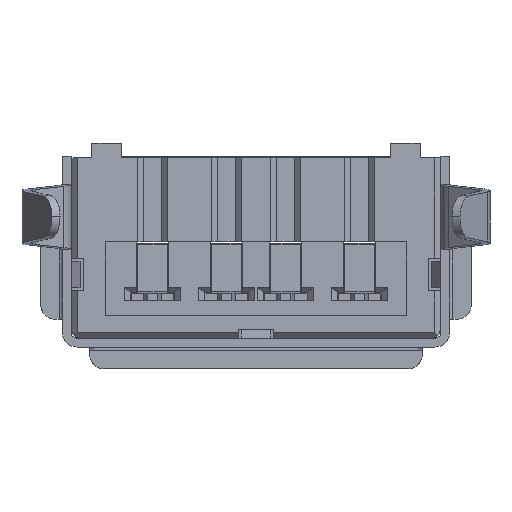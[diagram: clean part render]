
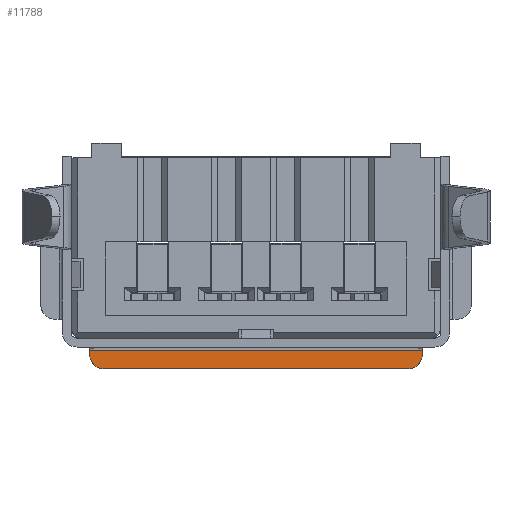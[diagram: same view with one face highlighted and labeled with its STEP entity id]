
A CAD part, front view. The second image highlights one B-rep face of the part: STEP entity #11788.
In plain terms, the highlighted planar face has unit normal (0, -1, 0).
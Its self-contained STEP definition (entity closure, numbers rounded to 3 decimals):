
#174 = CARTESIAN_POINT ( 'NONE',  ( 5.625, 6.85, 0. ) ) ;
#301 = VECTOR ( 'NONE', #9829, 1000. ) ;
#624 = VECTOR ( 'NONE', #3200, 1000. ) ;
#785 = AXIS2_PLACEMENT_3D ( 'NONE', #11261, #17445, #7973 ) ;
#992 = VERTEX_POINT ( 'NONE', #19504 ) ;
#1148 = CARTESIAN_POINT ( 'NONE',  ( -5.625, 6.85, -0.4 ) ) ;
#2433 = AXIS2_PLACEMENT_3D ( 'NONE', #8808, #13946, #12000 ) ;
#2630 = VERTEX_POINT ( 'NONE', #15059 ) ;
#3095 = LINE ( 'NONE', #17503, #624 ) ;
#3200 = DIRECTION ( 'NONE',  ( 1., 0., 0. ) ) ;
#3764 = CIRCLE ( 'NONE', #17918, 0.5 ) ;
#3880 = VECTOR ( 'NONE', #15398, 1000. ) ;
#4156 = ORIENTED_EDGE ( 'NONE', *, *, #19806, .T. ) ;
#4243 = EDGE_CURVE ( 'NONE', #11407, #992, #13577, .T. ) ;
#4872 = VERTEX_POINT ( 'NONE', #6754 ) ;
#5032 = DIRECTION ( 'NONE',  ( 0., -1., 0. ) ) ;
#5617 = EDGE_CURVE ( 'NONE', #4872, #19357, #3095, .T. ) ;
#5754 = DIRECTION ( 'NONE',  ( 0., 0., -1. ) ) ;
#5923 = VERTEX_POINT ( 'NONE', #6141 ) ;
#6001 = EDGE_CURVE ( 'NONE', #5923, #2630, #6344, .T. ) ;
#6004 = ORIENTED_EDGE ( 'NONE', *, *, #12941, .T. ) ;
#6141 = CARTESIAN_POINT ( 'NONE',  ( 5.625, 6.85, -0.54 ) ) ;
#6344 = LINE ( 'NONE', #174, #301 ) ;
#6754 = CARTESIAN_POINT ( 'NONE',  ( -5.125, 6.85, -1.04 ) ) ;
#7274 = PLANE ( 'NONE',  #2433 ) ;
#7476 = LINE ( 'NONE', #13750, #3880 ) ;
#7679 = CIRCLE ( 'NONE', #785, 0.5 ) ;
#7973 = DIRECTION ( 'NONE',  ( 0., 0., -1. ) ) ;
#8808 = CARTESIAN_POINT ( 'NONE',  ( 0., 6.85, 0. ) ) ;
#8952 = EDGE_CURVE ( 'NONE', #19357, #5923, #3764, .T. ) ;
#9829 = DIRECTION ( 'NONE',  ( 0., 0., 1. ) ) ;
#10246 = ORIENTED_EDGE ( 'NONE', *, *, #6001, .T. ) ;
#11261 = CARTESIAN_POINT ( 'NONE',  ( -5.125, 6.85, -0.54 ) ) ;
#11407 = VERTEX_POINT ( 'NONE', #1148 ) ;
#11788 = ADVANCED_FACE ( 'NONE', ( #18678 ), #7274, .T. ) ;
#11908 = VECTOR ( 'NONE', #5754, 1000. ) ;
#12000 = DIRECTION ( 'NONE',  ( 0., 0., -1. ) ) ;
#12529 = CARTESIAN_POINT ( 'NONE',  ( 5.125, 6.85, -1.04 ) ) ;
#12766 = CARTESIAN_POINT ( 'NONE',  ( 5.125, 6.85, -0.54 ) ) ;
#12941 = EDGE_CURVE ( 'NONE', #2630, #11407, #7476, .T. ) ;
#13577 = LINE ( 'NONE', #19847, #11908 ) ;
#13750 = CARTESIAN_POINT ( 'NONE',  ( 5.625, 6.85, -0.4 ) ) ;
#13946 = DIRECTION ( 'NONE',  ( 0., -1., 0. ) ) ;
#15059 = CARTESIAN_POINT ( 'NONE',  ( 5.625, 6.85, -0.4 ) ) ;
#15398 = DIRECTION ( 'NONE',  ( -1., 0., 0. ) ) ;
#17445 = DIRECTION ( 'NONE',  ( 0., -1., 0. ) ) ;
#17503 = CARTESIAN_POINT ( 'NONE',  ( 0., 6.85, -1.04 ) ) ;
#17706 = DIRECTION ( 'NONE',  ( 0., 0., -1. ) ) ;
#17766 = ORIENTED_EDGE ( 'NONE', *, *, #4243, .T. ) ;
#17918 = AXIS2_PLACEMENT_3D ( 'NONE', #12766, #5032, #17706 ) ;
#18608 = ORIENTED_EDGE ( 'NONE', *, *, #8952, .T. ) ;
#18678 = FACE_OUTER_BOUND ( 'NONE', #19130, .T. ) ;
#19130 = EDGE_LOOP ( 'NONE', ( #4156, #20169, #18608, #10246, #6004, #17766 ) ) ;
#19357 = VERTEX_POINT ( 'NONE', #12529 ) ;
#19504 = CARTESIAN_POINT ( 'NONE',  ( -5.625, 6.85, -0.54 ) ) ;
#19806 = EDGE_CURVE ( 'NONE', #992, #4872, #7679, .T. ) ;
#19847 = CARTESIAN_POINT ( 'NONE',  ( -5.625, 6.85, 0. ) ) ;
#20169 = ORIENTED_EDGE ( 'NONE', *, *, #5617, .T. ) ;
